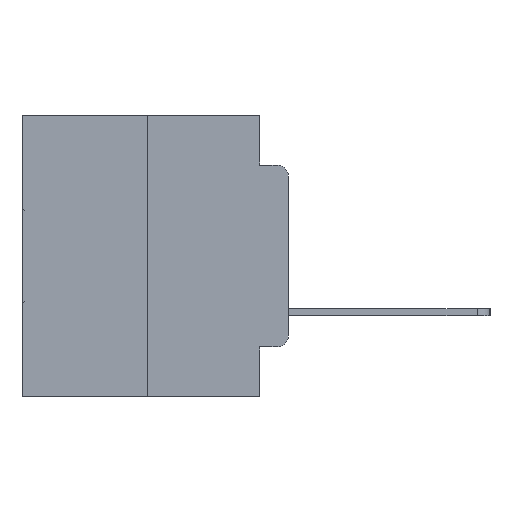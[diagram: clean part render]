
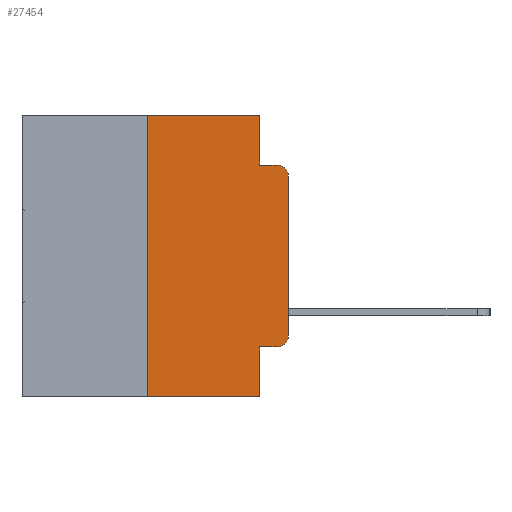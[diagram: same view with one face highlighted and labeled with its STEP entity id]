
A CAD part, left-side view. The second image highlights one B-rep face of the part: STEP entity #27454.
In plain terms, the highlighted planar face has unit normal (-1, 0, 0).
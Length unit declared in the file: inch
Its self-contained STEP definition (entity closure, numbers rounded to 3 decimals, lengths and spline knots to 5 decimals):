
#212 = CARTESIAN_POINT ( 'NONE',  ( 0., 0.25, -0.5 ) ) ;
#235 = VECTOR ( 'NONE', #28296, 39.37008 ) ;
#252 = CARTESIAN_POINT ( 'NONE',  ( 0., 0.051, -0.5 ) ) ;
#573 = LINE ( 'NONE', #1615, #29774 ) ;
#1187 = ORIENTED_EDGE ( 'NONE', *, *, #28690, .F. ) ;
#1568 = ORIENTED_EDGE ( 'NONE', *, *, #29185, .F. ) ;
#1615 = CARTESIAN_POINT ( 'NONE',  ( 0., 0., 0. ) ) ;
#2077 = DIRECTION ( 'NONE',  ( 0., 0., -1. ) ) ;
#2497 = LINE ( 'NONE', #24130, #14374 ) ;
#4228 = LINE ( 'NONE', #13670, #16124 ) ;
#4377 = LINE ( 'NONE', #7096, #21830 ) ;
#4568 = DIRECTION ( 'NONE',  ( 0., -1., 0. ) ) ;
#4618 = VECTOR ( 'NONE', #29917, 39.37008 ) ;
#4630 = LINE ( 'NONE', #15930, #28306 ) ;
#4816 = VERTEX_POINT ( 'NONE', #10463 ) ;
#5287 = VERTEX_POINT ( 'NONE', #26597 ) ;
#5525 = EDGE_CURVE ( 'NONE', #4816, #28549, #573, .T. ) ;
#6852 = CARTESIAN_POINT ( 'NONE',  ( 0., 0., -0.1085 ) ) ;
#6890 = EDGE_CURVE ( 'NONE', #20054, #4816, #27997, .T. ) ;
#7096 = CARTESIAN_POINT ( 'NONE',  ( 0., 0.25, 0. ) ) ;
#7307 = CARTESIAN_POINT ( 'NONE',  ( 0., 0.473, 0. ) ) ;
#9085 = EDGE_CURVE ( 'NONE', #13972, #20054, #16066, .T. ) ;
#9390 = ORIENTED_EDGE ( 'NONE', *, *, #9085, .T. ) ;
#10463 = CARTESIAN_POINT ( 'NONE',  ( 0., 0., -0.3915 ) ) ;
#11433 = DIRECTION ( 'NONE',  ( -1., 0., 0. ) ) ;
#11903 = AXIS2_PLACEMENT_3D ( 'NONE', #7307, #28569, #14473 ) ;
#12086 = PLANE ( 'NONE',  #11903 ) ;
#12806 = CARTESIAN_POINT ( 'NONE',  ( 0., 0.051, -0.0885 ) ) ;
#13592 = VERTEX_POINT ( 'NONE', #212 ) ;
#13670 = CARTESIAN_POINT ( 'NONE',  ( 0., 0.051, 0. ) ) ;
#13972 = VERTEX_POINT ( 'NONE', #20401 ) ;
#14021 = EDGE_CURVE ( 'NONE', #13592, #28010, #29030, .T. ) ;
#14374 = VECTOR ( 'NONE', #26505, 39.37008 ) ;
#14473 = DIRECTION ( 'NONE',  ( 0., 0., -1. ) ) ;
#15930 = CARTESIAN_POINT ( 'NONE',  ( 0., 0.473, 0. ) ) ;
#16066 = LINE ( 'NONE', #28352, #27859 ) ;
#16068 = DIRECTION ( 'NONE',  ( 0., 0., -1. ) ) ;
#16124 = VECTOR ( 'NONE', #16068, 39.37008 ) ;
#16279 = DIRECTION ( 'NONE',  ( -1., 0., 0. ) ) ;
#16462 = VERTEX_POINT ( 'NONE', #12806 ) ;
#16550 = DIRECTION ( 'NONE',  ( 0., 0., 1. ) ) ;
#16804 = ORIENTED_EDGE ( 'NONE', *, *, #19438, .F. ) ;
#17189 = CARTESIAN_POINT ( 'NONE',  ( 0., 0.051, 0. ) ) ;
#17721 = AXIS2_PLACEMENT_3D ( 'NONE', #30357, #16279, #2077 ) ;
#18118 = EDGE_CURVE ( 'NONE', #13592, #5287, #4377, .T. ) ;
#18283 = ORIENTED_EDGE ( 'NONE', *, *, #14021, .T. ) ;
#18316 = DIRECTION ( 'NONE',  ( 0., -1., 0. ) ) ;
#18624 = EDGE_CURVE ( 'NONE', #28549, #19271, #20325, .T. ) ;
#19167 = LINE ( 'NONE', #25942, #235 ) ;
#19271 = VERTEX_POINT ( 'NONE', #20002 ) ;
#19438 = EDGE_CURVE ( 'NONE', #5287, #25162, #4630, .T. ) ;
#20002 = CARTESIAN_POINT ( 'NONE',  ( 0., 0.02, -0.0885 ) ) ;
#20054 = VERTEX_POINT ( 'NONE', #20553 ) ;
#20325 = CIRCLE ( 'NONE', #24938, 0.02 ) ;
#20401 = CARTESIAN_POINT ( 'NONE',  ( 0., 0.051, -0.4115 ) ) ;
#20498 = CARTESIAN_POINT ( 'NONE',  ( 0., 0.473, -0.5 ) ) ;
#20553 = CARTESIAN_POINT ( 'NONE',  ( 0., 0.02, -0.4115 ) ) ;
#20737 = EDGE_CURVE ( 'NONE', #25162, #16462, #4228, .T. ) ;
#21615 = ORIENTED_EDGE ( 'NONE', *, *, #20737, .F. ) ;
#21830 = VECTOR ( 'NONE', #16550, 39.37008 ) ;
#22932 = DIRECTION ( 'NONE',  ( 0., 0., 1. ) ) ;
#23414 = ORIENTED_EDGE ( 'NONE', *, *, #5525, .T. ) ;
#23450 = ORIENTED_EDGE ( 'NONE', *, *, #6890, .T. ) ;
#23724 = EDGE_LOOP ( 'NONE', ( #23414, #29655, #1187, #21615, #16804, #29311, #18283, #1568, #9390, #23450 ) ) ;
#24130 = CARTESIAN_POINT ( 'NONE',  ( 0., 0.051, -0.0885 ) ) ;
#24938 = AXIS2_PLACEMENT_3D ( 'NONE', #25572, #11433, #27934 ) ;
#25162 = VERTEX_POINT ( 'NONE', #17189 ) ;
#25524 = FACE_OUTER_BOUND ( 'NONE', #23724, .T. ) ;
#25572 = CARTESIAN_POINT ( 'NONE',  ( 0., 0.02, -0.1085 ) ) ;
#25942 = CARTESIAN_POINT ( 'NONE',  ( 0., 0.051, 0. ) ) ;
#26505 = DIRECTION ( 'NONE',  ( 0., -1., 0. ) ) ;
#26597 = CARTESIAN_POINT ( 'NONE',  ( 0., 0.25, 0. ) ) ;
#27454 = ADVANCED_FACE ( 'NONE', ( #25524 ), #12086, .F. ) ;
#27859 = VECTOR ( 'NONE', #4568, 39.37008 ) ;
#27934 = DIRECTION ( 'NONE',  ( 0., 0., -1. ) ) ;
#27997 = CIRCLE ( 'NONE', #17721, 0.02 ) ;
#28010 = VERTEX_POINT ( 'NONE', #252 ) ;
#28296 = DIRECTION ( 'NONE',  ( 0., 0., -1. ) ) ;
#28306 = VECTOR ( 'NONE', #18316, 39.37008 ) ;
#28352 = CARTESIAN_POINT ( 'NONE',  ( 0., 0.051, -0.4115 ) ) ;
#28549 = VERTEX_POINT ( 'NONE', #6852 ) ;
#28569 = DIRECTION ( 'NONE',  ( 1., 0., 0. ) ) ;
#28690 = EDGE_CURVE ( 'NONE', #16462, #19271, #2497, .T. ) ;
#29030 = LINE ( 'NONE', #20498, #4618 ) ;
#29185 = EDGE_CURVE ( 'NONE', #13972, #28010, #19167, .T. ) ;
#29311 = ORIENTED_EDGE ( 'NONE', *, *, #18118, .F. ) ;
#29655 = ORIENTED_EDGE ( 'NONE', *, *, #18624, .T. ) ;
#29774 = VECTOR ( 'NONE', #22932, 39.37008 ) ;
#29917 = DIRECTION ( 'NONE',  ( 0., -1., 0. ) ) ;
#30357 = CARTESIAN_POINT ( 'NONE',  ( 0., 0.02, -0.3915 ) ) ;
